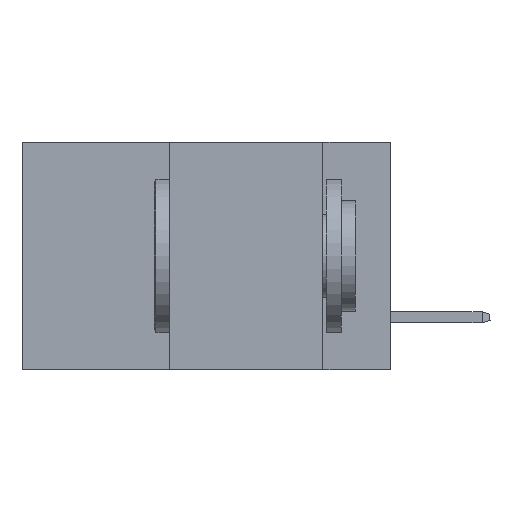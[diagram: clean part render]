
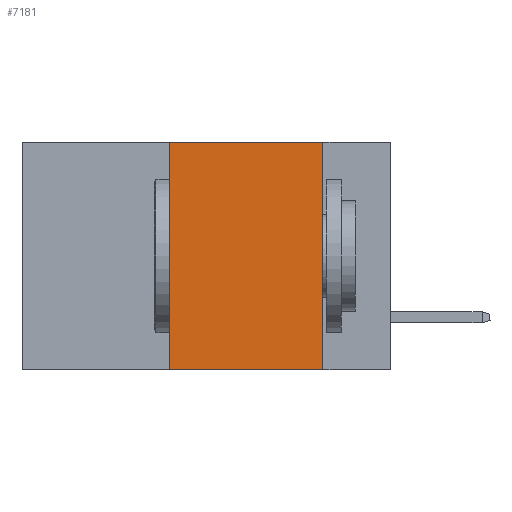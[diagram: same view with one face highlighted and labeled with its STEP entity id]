
A CAD part, left-side view. The second image highlights one B-rep face of the part: STEP entity #7181.
In plain terms, the highlighted planar face has unit normal (-1, 0, 0).
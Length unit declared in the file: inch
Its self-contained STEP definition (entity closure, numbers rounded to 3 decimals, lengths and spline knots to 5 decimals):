
#172 = VECTOR ( 'NONE', #3715, 39.37008 ) ;
#570 = DIRECTION ( 'NONE',  ( 0., 0., -1. ) ) ;
#573 = VECTOR ( 'NONE', #9227, 39.37008 ) ;
#2106 = EDGE_LOOP ( 'NONE', ( #5856, #2984, #7179, #4194 ) ) ;
#2637 = LINE ( 'NONE', #9200, #573 ) ;
#2984 = ORIENTED_EDGE ( 'NONE', *, *, #4696, .F. ) ;
#3011 = CARTESIAN_POINT ( 'NONE',  ( 0., 0.11, -0.37 ) ) ;
#3124 = EDGE_CURVE ( 'NONE', #4608, #7610, #4223, .T. ) ;
#3160 = EDGE_CURVE ( 'NONE', #4608, #8786, #7447, .T. ) ;
#3651 = FACE_OUTER_BOUND ( 'NONE', #2106, .T. ) ;
#3715 = DIRECTION ( 'NONE',  ( 0., 0., -1. ) ) ;
#3757 = CARTESIAN_POINT ( 'NONE',  ( 0., 0.11, 0. ) ) ;
#3833 = CARTESIAN_POINT ( 'NONE',  ( 0., 0.36, 0. ) ) ;
#3868 = DIRECTION ( 'NONE',  ( 0., 0., 1. ) ) ;
#4194 = ORIENTED_EDGE ( 'NONE', *, *, #3124, .T. ) ;
#4223 = LINE ( 'NONE', #6232, #10060 ) ;
#4608 = VERTEX_POINT ( 'NONE', #5908 ) ;
#4696 = EDGE_CURVE ( 'NONE', #8786, #6428, #2637, .T. ) ;
#4869 = VECTOR ( 'NONE', #3868, 39.37008 ) ;
#5357 = EDGE_CURVE ( 'NONE', #6428, #7610, #9285, .T. ) ;
#5561 = CARTESIAN_POINT ( 'NONE',  ( 0., 0.36, 0. ) ) ;
#5856 = ORIENTED_EDGE ( 'NONE', *, *, #5357, .F. ) ;
#5908 = CARTESIAN_POINT ( 'NONE',  ( 0., 0.36, -0.37 ) ) ;
#6232 = CARTESIAN_POINT ( 'NONE',  ( 0., 0.6, -0.37 ) ) ;
#6320 = DIRECTION ( 'NONE',  ( 0., -1., 0. ) ) ;
#6428 = VERTEX_POINT ( 'NONE', #6623 ) ;
#6623 = CARTESIAN_POINT ( 'NONE',  ( 0., 0.11, 0. ) ) ;
#6719 = CARTESIAN_POINT ( 'NONE',  ( 0., 0.6, 0. ) ) ;
#7179 = ORIENTED_EDGE ( 'NONE', *, *, #3160, .F. ) ;
#7181 = ADVANCED_FACE ( 'NONE', ( #3651 ), #9952, .F. ) ;
#7447 = LINE ( 'NONE', #3833, #4869 ) ;
#7610 = VERTEX_POINT ( 'NONE', #3011 ) ;
#8786 = VERTEX_POINT ( 'NONE', #5561 ) ;
#9200 = CARTESIAN_POINT ( 'NONE',  ( 0., 0.6, 0. ) ) ;
#9227 = DIRECTION ( 'NONE',  ( 0., -1., 0. ) ) ;
#9285 = LINE ( 'NONE', #3757, #172 ) ;
#9907 = DIRECTION ( 'NONE',  ( 1., 0., 0. ) ) ;
#9952 = PLANE ( 'NONE',  #10047 ) ;
#10047 = AXIS2_PLACEMENT_3D ( 'NONE', #6719, #9907, #570 ) ;
#10060 = VECTOR ( 'NONE', #6320, 39.37008 ) ;
